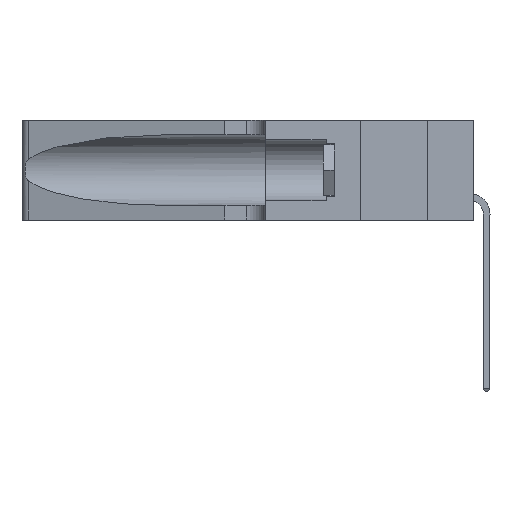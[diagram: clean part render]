
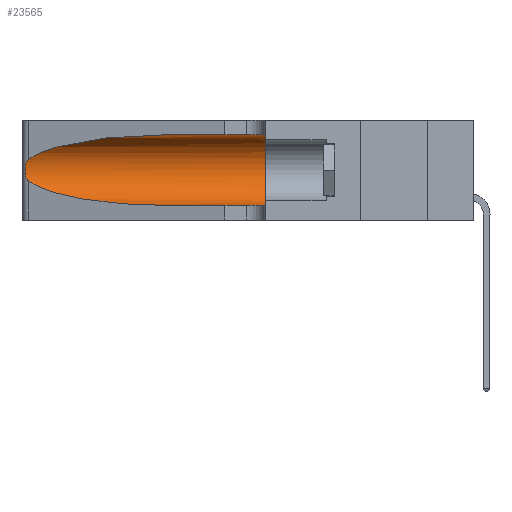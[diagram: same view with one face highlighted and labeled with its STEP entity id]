
A CAD part, left-side view. The second image highlights one B-rep face of the part: STEP entity #23565.
In plain terms, the highlighted cylindrical face has radius 3.308 mm (diameter 6.617 mm), a partial arc.
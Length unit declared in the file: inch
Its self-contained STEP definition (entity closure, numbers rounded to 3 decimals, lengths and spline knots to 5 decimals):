
#1305 = ORIENTED_EDGE ( 'NONE', *, *, #2720, .F. ) ;
#2092 = VERTEX_POINT ( 'NONE', #18025 ) ;
#2720 = EDGE_CURVE ( 'NONE', #11225, #38153, #7983, .T. ) ;
#3670 = CARTESIAN_POINT ( 'NONE',  ( 0.1305, 0.35, 0.185 ) ) ;
#4068 = CARTESIAN_POINT ( 'NONE',  ( 0.25487, 1.22718, 0.14631 ) ) ;
#5611 = CARTESIAN_POINT ( 'NONE',  ( 0.25639, 1.23186, 0.15144 ) ) ;
#5758 = ORIENTED_EDGE ( 'NONE', *, *, #25513, .T. ) ;
#7929 = VERTEX_POINT ( 'NONE', #33491 ) ;
#7983 = CIRCLE ( 'NONE', #28116, 0.13025 ) ;
#8133 = CARTESIAN_POINT ( 'NONE',  ( 0.25555, 1.22994, 0.2215 ) ) ;
#9074 = CARTESIAN_POINT ( 'NONE',  ( 0.1305, 0.72297, 0.31525 ) ) ;
#9162 = DIRECTION ( 'NONE',  ( 0., 0., 1. ) ) ;
#10520 = ORIENTED_EDGE ( 'NONE', *, *, #38965, .T. ) ;
#10992 = LINE ( 'NONE', #35552, #12396 ) ;
#11225 = VERTEX_POINT ( 'NONE', #13109 ) ;
#11331 =( BOUNDED_CURVE ( )  B_SPLINE_CURVE ( 3, ( #9074, #33477, #25174, #34269 ),
 .UNSPECIFIED., .F., .F. ) 
 B_SPLINE_CURVE_WITH_KNOTS ( ( 4, 4 ),
 ( 1.5708, 2.84003 ),
 .UNSPECIFIED. ) 
 CURVE ( )  GEOMETRIC_REPRESENTATION_ITEM ( )  RATIONAL_B_SPLINE_CURVE ( ( 1., 0.87, 0.87, 1. ) ) 
 REPRESENTATION_ITEM ( '' )  );
#11505 = VERTEX_POINT ( 'NONE', #25055 ) ;
#11663 = EDGE_CURVE ( 'NONE', #29695, #7929, #11331, .T. ) ;
#12158 = ORIENTED_EDGE ( 'NONE', *, *, #11663, .T. ) ;
#12396 = VECTOR ( 'NONE', #32029, 39.37008 ) ;
#13109 = CARTESIAN_POINT ( 'NONE',  ( 0.1305, 0.35, 0.31525 ) ) ;
#13696 = CARTESIAN_POINT ( 'NONE',  ( 0.25787, 1.23484, 0.2124 ) ) ;
#13989 = CARTESIAN_POINT ( 'NONE',  ( 0.1305, 1.61858, 0.05475 ) ) ;
#14103 = CARTESIAN_POINT ( 'NONE',  ( 0.25487, 1.22718, 0.22369 ) ) ;
#15512 = VECTOR ( 'NONE', #26250, 39.37008 ) ;
#16770 = CARTESIAN_POINT ( 'NONE',  ( 0.25854, 1.2359, 0.20912 ) ) ;
#17292 = EDGE_CURVE ( 'NONE', #29695, #11225, #10992, .T. ) ;
#17574 = CARTESIAN_POINT ( 'NONE',  ( 0.25856, 1.23593, 0.16098 ) ) ;
#17642 = AXIS2_PLACEMENT_3D ( 'NONE', #30939, #19050, #28253 ) ;
#17981 = CARTESIAN_POINT ( 'NONE',  ( 0.26017, 1.23833, 0.17102 ) ) ;
#18025 = CARTESIAN_POINT ( 'NONE',  ( 0.25487, 1.22718, 0.14631 ) ) ;
#19050 = DIRECTION ( 'NONE',  ( 0., -1., 0. ) ) ;
#19833 = CARTESIAN_POINT ( 'NONE',  ( 0.26075, 1.23896, 0.19203 ) ) ;
#20481 = CARTESIAN_POINT ( 'NONE',  ( 0.26075, 1.23896, 0.178 ) ) ;
#20763 = EDGE_CURVE ( 'NONE', #2092, #11505, #36783, .T. ) ;
#20863 = CARTESIAN_POINT ( 'NONE',  ( 0.25555, 1.22993, 0.14849 ) ) ;
#23239 = FACE_OUTER_BOUND ( 'NONE', #32157, .T. ) ;
#23565 = ADVANCED_FACE ( 'NONE', ( #23239 ), #24204, .F. ) ;
#24204 = CYLINDRICAL_SURFACE ( 'NONE', #17642, 0.13025 ) ;
#25055 = CARTESIAN_POINT ( 'NONE',  ( 0.1305, 0.72297, 0.05475 ) ) ;
#25174 = CARTESIAN_POINT ( 'NONE',  ( 0.2373, 1.15595, 0.28018 ) ) ;
#25513 = EDGE_CURVE ( 'NONE', #11505, #38153, #27440, .T. ) ;
#26250 = DIRECTION ( 'NONE',  ( 0., -1., 0. ) ) ;
#27440 = LINE ( 'NONE', #13989, #15512 ) ;
#27790 = DIRECTION ( 'NONE',  ( 0., 1., 0. ) ) ;
#28116 = AXIS2_PLACEMENT_3D ( 'NONE', #3670, #27790, #9162 ) ;
#28253 = DIRECTION ( 'NONE',  ( 0., 0., -1. ) ) ;
#28527 = ORIENTED_EDGE ( 'NONE', *, *, #20763, .T. ) ;
#28948 = B_SPLINE_CURVE_WITH_KNOTS ( 'NONE', 3,
 ( #14103, #8133, #29450, #13696, #16770, #38145, #19833, #20481, #17981, #17574, #32778, #5611, #20863, #35751 ),
 .UNSPECIFIED., .F., .F.,
 ( 4, 2, 2, 2, 2, 2, 4 ),
 ( 0., 0.00027, 0.00053, 0.00107, 0.0016, 0.00187, 0.00214 ),
 .UNSPECIFIED. ) ;
#29116 = CARTESIAN_POINT ( 'NONE',  ( 0.1305, 0.72297, 0.05475 ) ) ;
#29450 = CARTESIAN_POINT ( 'NONE',  ( 0.25639, 1.23184, 0.21858 ) ) ;
#29695 = VERTEX_POINT ( 'NONE', #30035 ) ;
#30035 = CARTESIAN_POINT ( 'NONE',  ( 0.1305, 0.72297, 0.31525 ) ) ;
#30939 = CARTESIAN_POINT ( 'NONE',  ( 0.1305, 1.61858, 0.185 ) ) ;
#31641 = CARTESIAN_POINT ( 'NONE',  ( 0.2373, 1.15595, 0.08982 ) ) ;
#32029 = DIRECTION ( 'NONE',  ( 0., -1., 0. ) ) ;
#32157 = EDGE_LOOP ( 'NONE', ( #12158, #10520, #28527, #5758, #1305, #36356 ) ) ;
#32778 = CARTESIAN_POINT ( 'NONE',  ( 0.25789, 1.23486, 0.15765 ) ) ;
#33477 = CARTESIAN_POINT ( 'NONE',  ( 0.18966, 0.96281, 0.31525 ) ) ;
#33491 = CARTESIAN_POINT ( 'NONE',  ( 0.25487, 1.22718, 0.22369 ) ) ;
#34269 = CARTESIAN_POINT ( 'NONE',  ( 0.25487, 1.22718, 0.22369 ) ) ;
#34613 = CARTESIAN_POINT ( 'NONE',  ( 0.1305, 0.35, 0.05475 ) ) ;
#35030 = CARTESIAN_POINT ( 'NONE',  ( 0.18966, 0.96281, 0.05475 ) ) ;
#35552 = CARTESIAN_POINT ( 'NONE',  ( 0.1305, 1.61858, 0.31525 ) ) ;
#35751 = CARTESIAN_POINT ( 'NONE',  ( 0.25487, 1.22718, 0.14631 ) ) ;
#36356 = ORIENTED_EDGE ( 'NONE', *, *, #17292, .F. ) ;
#36783 =( BOUNDED_CURVE ( )  B_SPLINE_CURVE ( 3, ( #4068, #31641, #35030, #29116 ),
 .UNSPECIFIED., .F., .F. ) 
 B_SPLINE_CURVE_WITH_KNOTS ( ( 4, 4 ),
 ( 3.44316, 4.71239 ),
 .UNSPECIFIED. ) 
 CURVE ( )  GEOMETRIC_REPRESENTATION_ITEM ( )  RATIONAL_B_SPLINE_CURVE ( ( 1., 0.87, 0.87, 1. ) ) 
 REPRESENTATION_ITEM ( '' )  );
#38145 = CARTESIAN_POINT ( 'NONE',  ( 0.26018, 1.23835, 0.19895 ) ) ;
#38153 = VERTEX_POINT ( 'NONE', #34613 ) ;
#38965 = EDGE_CURVE ( 'NONE', #7929, #2092, #28948, .T. ) ;
